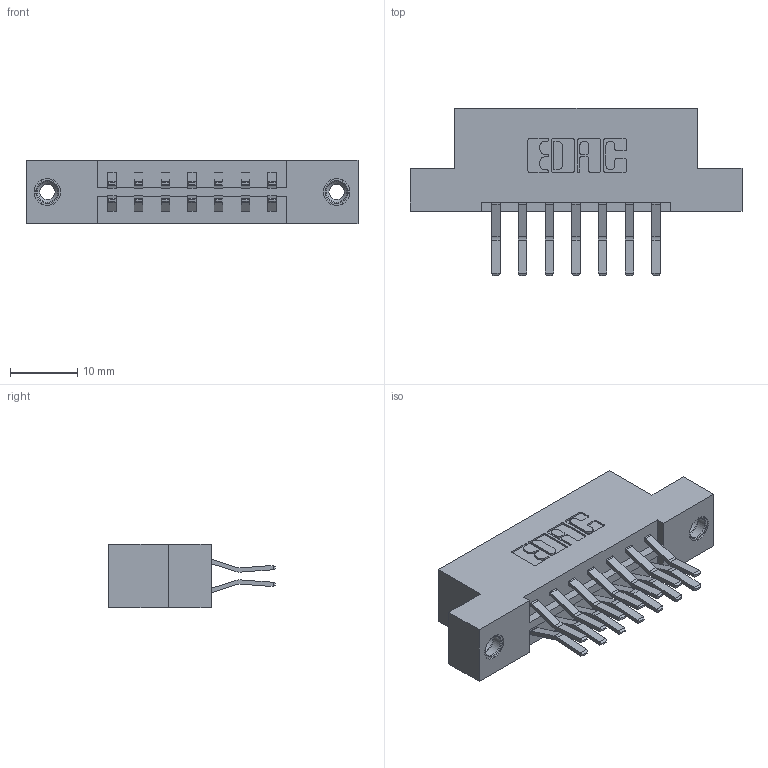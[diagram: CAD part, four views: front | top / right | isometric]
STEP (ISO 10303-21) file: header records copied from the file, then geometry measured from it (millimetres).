
FILE_DESCRIPTION (( 'STEP AP203' ), '1' );
FILE_NAME ('833-014-560-208.STEP', '2020-05-31T15:16:18', ( '' ), ( '' ), 'SwSTEP 2.0', 'SolidWorks 2020', '' );
FILE_SCHEMA (( 'CONFIG_CONTROL_DESIGN' ));
Length unit declared in the file: inch
Products named in the file (4): 833 Part_Flush - .156 Dia - TI; 345-250-001_345-250-003-102; 345-292-001_560 Tail; 833-014-560-208
Assembly tree (17 placements, depth 2):
  833-014-560-208
    833 Part_Flush - .156 Dia - TI
    345-292-001_560 Tail  x14
    345-250-001_345-250-003-102  x2
Bounding box: 49.28 x 24.78 x 9.4 mm (x, y, z)
Volume: 4788.7 mm3; surface area: 5568.9 mm2
Topology: 17 solids, 17 shells, 930 faces, 2701 edges, 1774 vertices
Faces by surface type: plane 606, cylinder 308, cone 12, torus 4
Entity records: 10304 total; most frequent: CARTESIAN_POINT 1733, ORIENTED_EDGE 1662, DIRECTION 1577, EDGE_CURVE 831, LINE 679, VECTOR 679, VERTEX_POINT 548, AXIS2_PLACEMENT_3D 449
